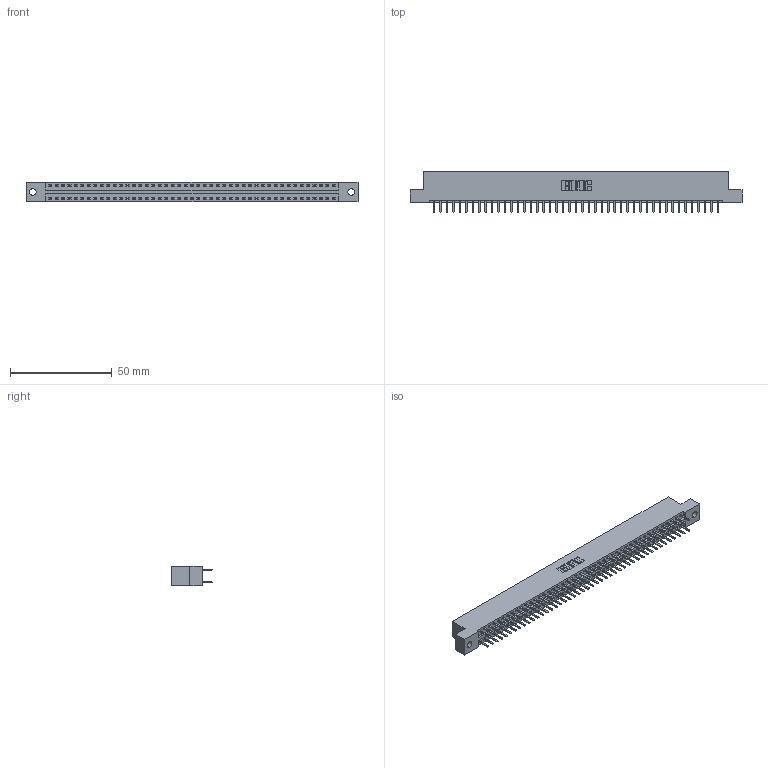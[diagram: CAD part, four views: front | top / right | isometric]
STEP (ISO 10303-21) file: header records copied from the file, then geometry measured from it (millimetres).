
FILE_DESCRIPTION (( 'STEP AP203' ), '1' );
FILE_NAME ('346-090-520-202.STEP', '2018-08-30T01:17:14', ( '' ), ( '' ), 'SwSTEP 2.0', 'SolidWorks 2016', '' );
FILE_SCHEMA (( 'CONFIG_CONTROL_DESIGN' ));
Length unit declared in the file: inch
Products named in the file (3): 346 Part_Flush Mounting Lugs - 0.128 Dia; 345-292-001_345-293-120; 346-090-520-202
Assembly tree (91 placements, depth 2):
  346-090-520-202
    346 Part_Flush Mounting Lugs - 0.128 Dia
    345-292-001_345-293-120  x90
Bounding box: 163.45 x 20.02 x 9.4 mm (x, y, z)
Volume: 15885.4 mm3; surface area: 21520.7 mm2
Topology: 91 solids, 91 shells, 5162 faces, 14999 edges, 9758 vertices
Faces by surface type: plane 3406, cylinder 1756
Entity records: 29081 total; most frequent: CARTESIAN_POINT 4800, ORIENTED_EDGE 4722, DIRECTION 4269, EDGE_CURVE 2361, VECTOR 2045, LINE 2045, VERTEX_POINT 1570, AXIS2_PLACEMENT_3D 1112
